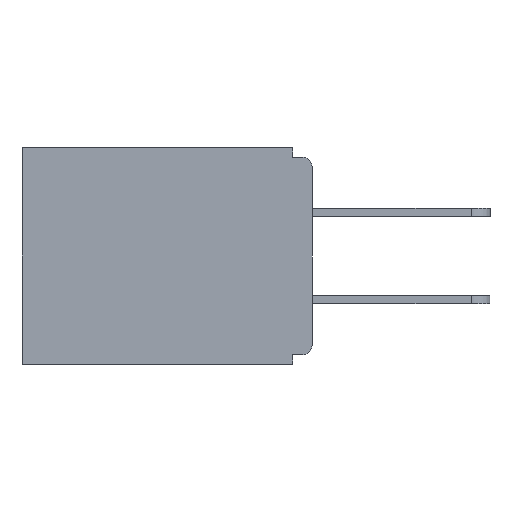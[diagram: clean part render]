
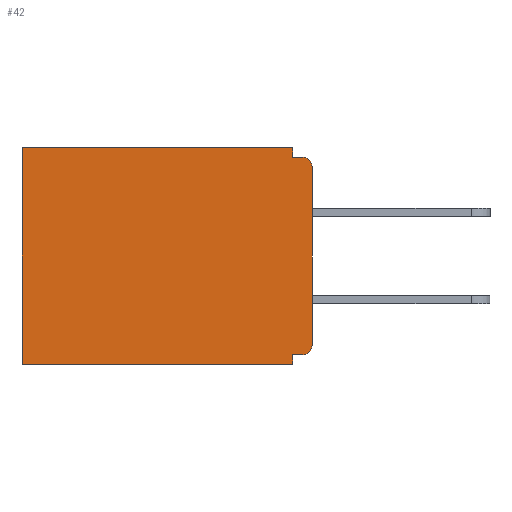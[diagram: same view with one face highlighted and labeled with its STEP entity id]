
A CAD part, left-side view. The second image highlights one B-rep face of the part: STEP entity #42.
In plain terms, the highlighted planar face has unit normal (-1, 0, 0).
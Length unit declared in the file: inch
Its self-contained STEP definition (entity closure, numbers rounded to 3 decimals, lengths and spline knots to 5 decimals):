
#42 = ADVANCED_FACE ( 'NONE', ( #2903 ), #3496, .F. ) ;
#44 = ORIENTED_EDGE ( 'NONE', *, *, #9804, .F. ) ;
#52 = DIRECTION ( 'NONE',  ( 0., 1., 0. ) ) ;
#113 = CARTESIAN_POINT ( 'NONE',  ( 0.298, 0.031, 0. ) ) ;
#278 = DIRECTION ( 'NONE',  ( 0., 0., -1. ) ) ;
#582 = ORIENTED_EDGE ( 'NONE', *, *, #11853, .F. ) ;
#640 = VERTEX_POINT ( 'NONE', #12238 ) ;
#1099 = EDGE_CURVE ( 'NONE', #7061, #12310, #11843, .T. ) ;
#1288 = VECTOR ( 'NONE', #1628, 39.37008 ) ;
#1628 = DIRECTION ( 'NONE',  ( 0., 0., -1. ) ) ;
#1643 = DIRECTION ( 'NONE',  ( 0., 0., -1. ) ) ;
#1681 = EDGE_CURVE ( 'NONE', #640, #6736, #2571, .T. ) ;
#2075 = LINE ( 'NONE', #3755, #3717 ) ;
#2238 = VECTOR ( 'NONE', #1643, 39.37008 ) ;
#2354 = DIRECTION ( 'NONE',  ( -1., 0., 0. ) ) ;
#2518 = EDGE_LOOP ( 'NONE', ( #6602, #5680, #44, #7060, #8688, #6103, #7277, #582, #9827, #9543 ) ) ;
#2571 = LINE ( 'NONE', #4024, #8968 ) ;
#2645 = CARTESIAN_POINT ( 'NONE',  ( 0.298, 0.015, -0.328 ) ) ;
#2898 = VERTEX_POINT ( 'NONE', #12413 ) ;
#2903 = FACE_OUTER_BOUND ( 'NONE', #2518, .T. ) ;
#3217 = CARTESIAN_POINT ( 'NONE',  ( 0.298, 0., -0.03 ) ) ;
#3496 = PLANE ( 'NONE',  #4489 ) ;
#3618 = EDGE_CURVE ( 'NONE', #6285, #12310, #7674, .T. ) ;
#3717 = VECTOR ( 'NONE', #3999, 39.37008 ) ;
#3753 = EDGE_CURVE ( 'NONE', #8510, #640, #2075, .T. ) ;
#3755 = CARTESIAN_POINT ( 'NONE',  ( 0.298, 0., 0. ) ) ;
#3964 = CARTESIAN_POINT ( 'NONE',  ( 0.298, 0., -0.343 ) ) ;
#3999 = DIRECTION ( 'NONE',  ( 0., 1., 0. ) ) ;
#4024 = CARTESIAN_POINT ( 'NONE',  ( 0.298, 0.46, 0. ) ) ;
#4097 = LINE ( 'NONE', #6019, #7016 ) ;
#4130 = AXIS2_PLACEMENT_3D ( 'NONE', #10323, #2354, #11079 ) ;
#4150 = VERTEX_POINT ( 'NONE', #5103 ) ;
#4479 = CARTESIAN_POINT ( 'NONE',  ( 0.298, 0.031, -0.343 ) ) ;
#4489 = AXIS2_PLACEMENT_3D ( 'NONE', #10280, #8407, #6646 ) ;
#4534 = CARTESIAN_POINT ( 'NONE',  ( 0.298, 0.031, -0.343 ) ) ;
#4776 = DIRECTION ( 'NONE',  ( 0., 0., -1. ) ) ;
#4937 = DIRECTION ( 'NONE',  ( 0., 1., 0. ) ) ;
#5103 = CARTESIAN_POINT ( 'NONE',  ( 0.298, 0.031, -0.343 ) ) ;
#5680 = ORIENTED_EDGE ( 'NONE', *, *, #7716, .F. ) ;
#5826 = DIRECTION ( 'NONE',  ( 0., -1., 0. ) ) ;
#5859 = LINE ( 'NONE', #4479, #1288 ) ;
#5930 = VECTOR ( 'NONE', #52, 39.37008 ) ;
#6019 = CARTESIAN_POINT ( 'NONE',  ( 0.298, 0., -0.015 ) ) ;
#6103 = ORIENTED_EDGE ( 'NONE', *, *, #7229, .F. ) ;
#6285 = VERTEX_POINT ( 'NONE', #2645 ) ;
#6328 = EDGE_CURVE ( 'NONE', #7061, #2898, #7956, .T. ) ;
#6602 = ORIENTED_EDGE ( 'NONE', *, *, #6328, .T. ) ;
#6646 = DIRECTION ( 'NONE',  ( 0., 0., -1. ) ) ;
#6736 = VERTEX_POINT ( 'NONE', #12329 ) ;
#6840 = CARTESIAN_POINT ( 'NONE',  ( 0.298, 0., -0.328 ) ) ;
#7016 = VECTOR ( 'NONE', #5826, 39.37008 ) ;
#7060 = ORIENTED_EDGE ( 'NONE', *, *, #3753, .T. ) ;
#7061 = VERTEX_POINT ( 'NONE', #3217 ) ;
#7107 = LINE ( 'NONE', #4534, #2238 ) ;
#7229 = EDGE_CURVE ( 'NONE', #4150, #6736, #8546, .T. ) ;
#7277 = ORIENTED_EDGE ( 'NONE', *, *, #10005, .F. ) ;
#7505 = VERTEX_POINT ( 'NONE', #8808 ) ;
#7674 = CIRCLE ( 'NONE', #8297, 0.015 ) ;
#7716 = EDGE_CURVE ( 'NONE', #7505, #2898, #4097, .T. ) ;
#7956 = CIRCLE ( 'NONE', #4130, 0.015 ) ;
#8108 = CARTESIAN_POINT ( 'NONE',  ( 0.298, 0.031, -0.328 ) ) ;
#8213 = VERTEX_POINT ( 'NONE', #8108 ) ;
#8297 = AXIS2_PLACEMENT_3D ( 'NONE', #8712, #10636, #10591 ) ;
#8335 = CARTESIAN_POINT ( 'NONE',  ( 0.298, 0., -0.313 ) ) ;
#8407 = DIRECTION ( 'NONE',  ( 1., 0., 0. ) ) ;
#8510 = VERTEX_POINT ( 'NONE', #113 ) ;
#8546 = LINE ( 'NONE', #3964, #12293 ) ;
#8688 = ORIENTED_EDGE ( 'NONE', *, *, #1681, .T. ) ;
#8712 = CARTESIAN_POINT ( 'NONE',  ( 0.298, 0.015, -0.313 ) ) ;
#8808 = CARTESIAN_POINT ( 'NONE',  ( 0.298, 0.031, -0.015 ) ) ;
#8827 = LINE ( 'NONE', #6840, #5930 ) ;
#8835 = VECTOR ( 'NONE', #4776, 39.37008 ) ;
#8968 = VECTOR ( 'NONE', #278, 39.37008 ) ;
#9543 = ORIENTED_EDGE ( 'NONE', *, *, #1099, .F. ) ;
#9804 = EDGE_CURVE ( 'NONE', #8510, #7505, #7107, .T. ) ;
#9827 = ORIENTED_EDGE ( 'NONE', *, *, #3618, .T. ) ;
#10005 = EDGE_CURVE ( 'NONE', #8213, #4150, #5859, .T. ) ;
#10280 = CARTESIAN_POINT ( 'NONE',  ( 0.298, 0., 0. ) ) ;
#10323 = CARTESIAN_POINT ( 'NONE',  ( 0.298, 0.015, -0.03 ) ) ;
#10591 = DIRECTION ( 'NONE',  ( 0., 0., -1. ) ) ;
#10636 = DIRECTION ( 'NONE',  ( -1., 0., 0. ) ) ;
#11079 = DIRECTION ( 'NONE',  ( 0., 0., -1. ) ) ;
#11843 = LINE ( 'NONE', #12431, #8835 ) ;
#11853 = EDGE_CURVE ( 'NONE', #6285, #8213, #8827, .T. ) ;
#12238 = CARTESIAN_POINT ( 'NONE',  ( 0.298, 0.46, 0. ) ) ;
#12293 = VECTOR ( 'NONE', #4937, 39.37008 ) ;
#12310 = VERTEX_POINT ( 'NONE', #8335 ) ;
#12329 = CARTESIAN_POINT ( 'NONE',  ( 0.298, 0.46, -0.343 ) ) ;
#12413 = CARTESIAN_POINT ( 'NONE',  ( 0.298, 0.015, -0.015 ) ) ;
#12431 = CARTESIAN_POINT ( 'NONE',  ( 0.298, 0., 0. ) ) ;
